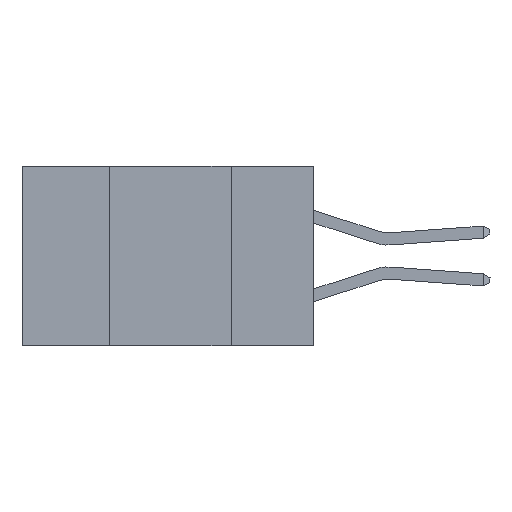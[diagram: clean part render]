
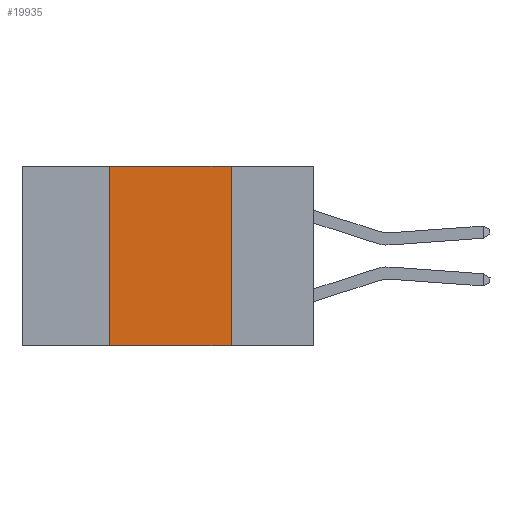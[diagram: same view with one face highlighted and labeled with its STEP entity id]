
A CAD part, left-side view. The second image highlights one B-rep face of the part: STEP entity #19935.
In plain terms, the highlighted planar face has unit normal (-1, 0, 0).
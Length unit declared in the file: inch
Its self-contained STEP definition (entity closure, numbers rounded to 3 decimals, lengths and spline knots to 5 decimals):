
#939 = VERTEX_POINT ( 'NONE', #3239 ) ;
#948 = LINE ( 'NONE', #10142, #10337 ) ;
#2793 = EDGE_CURVE ( 'NONE', #939, #5225, #19067, .T. ) ;
#3074 = DIRECTION ( 'NONE',  ( 0., 0., -1. ) ) ;
#3239 = CARTESIAN_POINT ( 'NONE',  ( 0., 0.17, 0. ) ) ;
#3526 = AXIS2_PLACEMENT_3D ( 'NONE', #7260, #20084, #9148 ) ;
#3548 = PLANE ( 'NONE',  #3526 ) ;
#3721 = ORIENTED_EDGE ( 'NONE', *, *, #11506, .T. ) ;
#3875 = VECTOR ( 'NONE', #3074, 39.37008 ) ;
#4593 = EDGE_LOOP ( 'NONE', ( #11813, #16677, #22057, #3721 ) ) ;
#4866 = VERTEX_POINT ( 'NONE', #19844 ) ;
#4994 = LINE ( 'NONE', #10127, #18501 ) ;
#5225 = VERTEX_POINT ( 'NONE', #9862 ) ;
#7260 = CARTESIAN_POINT ( 'NONE',  ( 0., 0.6, 0. ) ) ;
#8623 = CARTESIAN_POINT ( 'NONE',  ( 0., 0.42, -0.37 ) ) ;
#9148 = DIRECTION ( 'NONE',  ( 0., 0., -1. ) ) ;
#9862 = CARTESIAN_POINT ( 'NONE',  ( 0., 0.17, -0.37 ) ) ;
#10127 = CARTESIAN_POINT ( 'NONE',  ( 0., 0.6, -0.37 ) ) ;
#10142 = CARTESIAN_POINT ( 'NONE',  ( 0., 0.6, 0. ) ) ;
#10337 = VECTOR ( 'NONE', #11966, 39.37008 ) ;
#11506 = EDGE_CURVE ( 'NONE', #13333, #5225, #4994, .T. ) ;
#11813 = ORIENTED_EDGE ( 'NONE', *, *, #2793, .F. ) ;
#11966 = DIRECTION ( 'NONE',  ( 0., -1., 0. ) ) ;
#12212 = CARTESIAN_POINT ( 'NONE',  ( 0., 0.17, 0. ) ) ;
#12752 = EDGE_CURVE ( 'NONE', #13333, #4866, #19585, .T. ) ;
#13333 = VERTEX_POINT ( 'NONE', #8623 ) ;
#16677 = ORIENTED_EDGE ( 'NONE', *, *, #19647, .F. ) ;
#18501 = VECTOR ( 'NONE', #21027, 39.37008 ) ;
#19067 = LINE ( 'NONE', #12212, #3875 ) ;
#19585 = LINE ( 'NONE', #21491, #23804 ) ;
#19647 = EDGE_CURVE ( 'NONE', #4866, #939, #948, .T. ) ;
#19844 = CARTESIAN_POINT ( 'NONE',  ( 0., 0.42, 0. ) ) ;
#19935 = ADVANCED_FACE ( 'NONE', ( #22807 ), #3548, .F. ) ;
#20084 = DIRECTION ( 'NONE',  ( 1., 0., 0. ) ) ;
#21027 = DIRECTION ( 'NONE',  ( 0., -1., 0. ) ) ;
#21491 = CARTESIAN_POINT ( 'NONE',  ( 0., 0.42, 0. ) ) ;
#22057 = ORIENTED_EDGE ( 'NONE', *, *, #12752, .F. ) ;
#22807 = FACE_OUTER_BOUND ( 'NONE', #4593, .T. ) ;
#23376 = DIRECTION ( 'NONE',  ( 0., 0., 1. ) ) ;
#23804 = VECTOR ( 'NONE', #23376, 39.37008 ) ;
